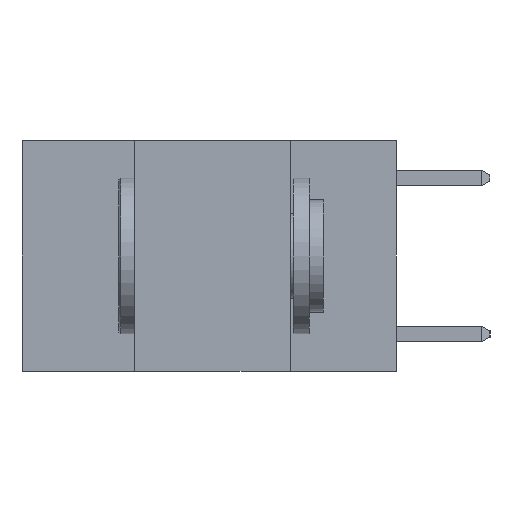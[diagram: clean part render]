
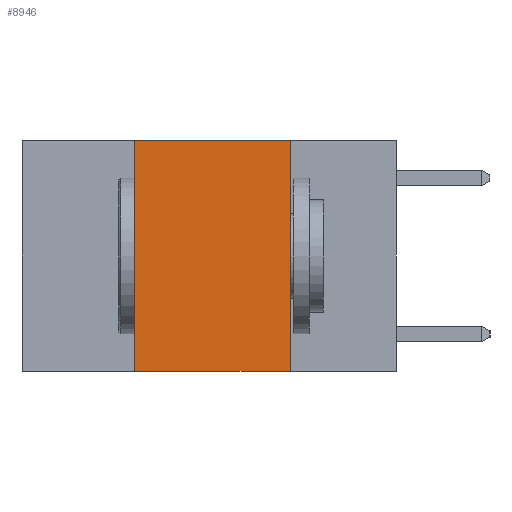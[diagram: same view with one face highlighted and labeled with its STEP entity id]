
A CAD part, left-side view. The second image highlights one B-rep face of the part: STEP entity #8946.
In plain terms, the highlighted planar face has unit normal (-1, 0, 0).
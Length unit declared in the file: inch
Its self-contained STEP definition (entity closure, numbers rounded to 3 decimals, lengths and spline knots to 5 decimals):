
#88 = VERTEX_POINT ( 'NONE', #2983 ) ;
#138 = EDGE_CURVE ( 'NONE', #2694, #88, #1572, .T. ) ;
#142 = VECTOR ( 'NONE', #966, 39.37008 ) ;
#175 = CARTESIAN_POINT ( 'NONE',  ( 0., 0.42, -0.37 ) ) ;
#283 = AXIS2_PLACEMENT_3D ( 'NONE', #4072, #10173, #4951 ) ;
#414 = LINE ( 'NONE', #2686, #142 ) ;
#431 = ORIENTED_EDGE ( 'NONE', *, *, #7512, .T. ) ;
#966 = DIRECTION ( 'NONE',  ( 0., -1., 0. ) ) ;
#1287 = ORIENTED_EDGE ( 'NONE', *, *, #138, .F. ) ;
#1572 = LINE ( 'NONE', #7769, #11150 ) ;
#2563 = VERTEX_POINT ( 'NONE', #7767 ) ;
#2686 = CARTESIAN_POINT ( 'NONE',  ( 0., 0.6, -0.37 ) ) ;
#2694 = VERTEX_POINT ( 'NONE', #175 ) ;
#2983 = CARTESIAN_POINT ( 'NONE',  ( 0., 0.42, 0. ) ) ;
#3703 = CARTESIAN_POINT ( 'NONE',  ( 0., 0.6, 0. ) ) ;
#4072 = CARTESIAN_POINT ( 'NONE',  ( 0., 0.6, 0. ) ) ;
#4264 = VECTOR ( 'NONE', #9812, 39.37008 ) ;
#4489 = CARTESIAN_POINT ( 'NONE',  ( 0., 0.17, 0. ) ) ;
#4538 = LINE ( 'NONE', #3703, #4264 ) ;
#4951 = DIRECTION ( 'NONE',  ( 0., 0., -1. ) ) ;
#5109 = FACE_OUTER_BOUND ( 'NONE', #6250, .T. ) ;
#5369 = DIRECTION ( 'NONE',  ( 0., 0., 1. ) ) ;
#5381 = DIRECTION ( 'NONE',  ( 0., 0., -1. ) ) ;
#5683 = EDGE_CURVE ( 'NONE', #6100, #2563, #6495, .T. ) ;
#6100 = VERTEX_POINT ( 'NONE', #7661 ) ;
#6250 = EDGE_LOOP ( 'NONE', ( #9331, #10495, #1287, #431 ) ) ;
#6495 = LINE ( 'NONE', #4489, #10874 ) ;
#7512 = EDGE_CURVE ( 'NONE', #2694, #2563, #414, .T. ) ;
#7661 = CARTESIAN_POINT ( 'NONE',  ( 0., 0.17, 0. ) ) ;
#7767 = CARTESIAN_POINT ( 'NONE',  ( 0., 0.17, -0.37 ) ) ;
#7769 = CARTESIAN_POINT ( 'NONE',  ( 0., 0.42, 0. ) ) ;
#8946 = ADVANCED_FACE ( 'NONE', ( #5109 ), #9303, .F. ) ;
#9303 = PLANE ( 'NONE',  #283 ) ;
#9331 = ORIENTED_EDGE ( 'NONE', *, *, #5683, .F. ) ;
#9812 = DIRECTION ( 'NONE',  ( 0., -1., 0. ) ) ;
#9898 = EDGE_CURVE ( 'NONE', #88, #6100, #4538, .T. ) ;
#10173 = DIRECTION ( 'NONE',  ( 1., 0., 0. ) ) ;
#10495 = ORIENTED_EDGE ( 'NONE', *, *, #9898, .F. ) ;
#10874 = VECTOR ( 'NONE', #5381, 39.37008 ) ;
#11150 = VECTOR ( 'NONE', #5369, 39.37008 ) ;
